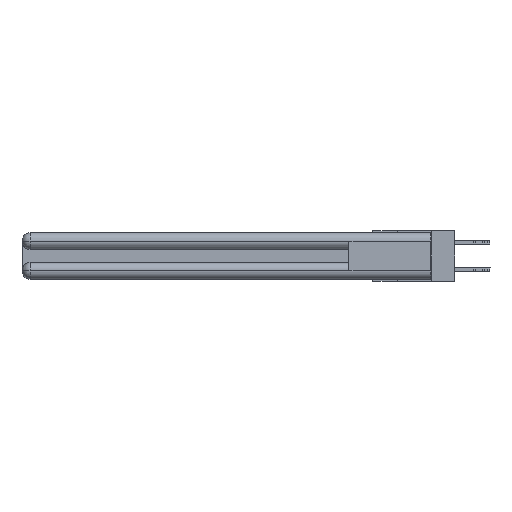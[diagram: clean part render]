
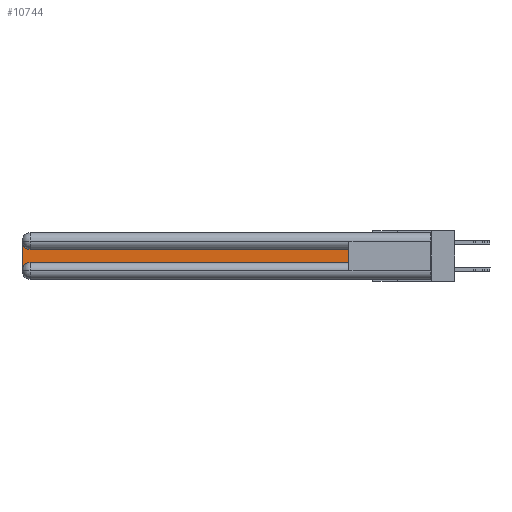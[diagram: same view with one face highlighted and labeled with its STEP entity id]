
A CAD part, left-side view. The second image highlights one B-rep face of the part: STEP entity #10744.
In plain terms, the highlighted planar face has unit normal (-1, 0, 0).
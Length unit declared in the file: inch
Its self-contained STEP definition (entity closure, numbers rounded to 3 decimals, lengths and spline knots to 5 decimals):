
#117 = LINE ( 'NONE', #29472, #9427 ) ;
#450 = EDGE_CURVE ( 'NONE', #2568, #6874, #19556, .T. ) ;
#1510 = CARTESIAN_POINT ( 'NONE',  ( 0.075, 0.6, -0.1225 ) ) ;
#2568 = VERTEX_POINT ( 'NONE', #13594 ) ;
#2750 = EDGE_LOOP ( 'NONE', ( #4872, #27061, #15855, #10406, #33133, #18451 ) ) ;
#3343 = DIRECTION ( 'NONE',  ( 0., -1., 0. ) ) ;
#4043 = DIRECTION ( 'NONE',  ( 1., 0., 0. ) ) ;
#4595 = AXIS2_PLACEMENT_3D ( 'NONE', #25945, #9605, #12233 ) ;
#4872 = ORIENTED_EDGE ( 'NONE', *, *, #20003, .T. ) ;
#6542 = LINE ( 'NONE', #30513, #8259 ) ;
#6874 = VERTEX_POINT ( 'NONE', #16815 ) ;
#7396 = DIRECTION ( 'NONE',  ( 0., 1., 0. ) ) ;
#7665 = EDGE_CURVE ( 'NONE', #16599, #8257, #28926, .T. ) ;
#8257 = VERTEX_POINT ( 'NONE', #32859 ) ;
#8259 = VECTOR ( 'NONE', #3343, 39.37008 ) ;
#9315 = CARTESIAN_POINT ( 'NONE',  ( 0.075, 0.6, -0.2175 ) ) ;
#9427 = VECTOR ( 'NONE', #32226, 39.37008 ) ;
#9605 = DIRECTION ( 'NONE',  ( 1., 0., 0. ) ) ;
#10406 = ORIENTED_EDGE ( 'NONE', *, *, #450, .T. ) ;
#10744 = ADVANCED_FACE ( 'NONE', ( #15960 ), #17992, .F. ) ;
#11776 = DIRECTION ( 'NONE',  ( 0., 0., -1. ) ) ;
#12233 = DIRECTION ( 'NONE',  ( 0., 0., -1. ) ) ;
#13594 = CARTESIAN_POINT ( 'NONE',  ( 0.075, 3., -0.2775 ) ) ;
#15482 = VERTEX_POINT ( 'NONE', #1510 ) ;
#15855 = ORIENTED_EDGE ( 'NONE', *, *, #17200, .T. ) ;
#15960 = FACE_OUTER_BOUND ( 'NONE', #2750, .T. ) ;
#16599 = VERTEX_POINT ( 'NONE', #23460 ) ;
#16815 = CARTESIAN_POINT ( 'NONE',  ( 0.075, 2.94, -0.2175 ) ) ;
#17200 = EDGE_CURVE ( 'NONE', #8257, #2568, #117, .T. ) ;
#17992 = PLANE ( 'NONE',  #4595 ) ;
#18451 = ORIENTED_EDGE ( 'NONE', *, *, #21430, .T. ) ;
#19099 = VECTOR ( 'NONE', #22168, 39.37008 ) ;
#19441 = CARTESIAN_POINT ( 'NONE',  ( 0.075, 0.6, -0.2175 ) ) ;
#19556 = CIRCLE ( 'NONE', #26095, 0.06 ) ;
#20003 = EDGE_CURVE ( 'NONE', #15482, #16599, #27233, .T. ) ;
#20514 = CARTESIAN_POINT ( 'NONE',  ( 0.075, 2.94, -0.0625 ) ) ;
#21430 = EDGE_CURVE ( 'NONE', #29503, #15482, #26272, .T. ) ;
#22168 = DIRECTION ( 'NONE',  ( 0., 0., 1. ) ) ;
#23002 = DIRECTION ( 'NONE',  ( 1., 0., 0. ) ) ;
#23460 = CARTESIAN_POINT ( 'NONE',  ( 0.075, 2.94, -0.1225 ) ) ;
#25945 = CARTESIAN_POINT ( 'NONE',  ( 0.075, 3., -0.1225 ) ) ;
#26095 = AXIS2_PLACEMENT_3D ( 'NONE', #33731, #23002, #11776 ) ;
#26272 = LINE ( 'NONE', #19441, #19099 ) ;
#26585 = CARTESIAN_POINT ( 'NONE',  ( 0.075, 0.6, -0.1225 ) ) ;
#27061 = ORIENTED_EDGE ( 'NONE', *, *, #7665, .T. ) ;
#27233 = LINE ( 'NONE', #26585, #27640 ) ;
#27608 = AXIS2_PLACEMENT_3D ( 'NONE', #20514, #4043, #28837 ) ;
#27640 = VECTOR ( 'NONE', #7396, 39.37008 ) ;
#28837 = DIRECTION ( 'NONE',  ( 0., 0., -1. ) ) ;
#28926 = CIRCLE ( 'NONE', #27608, 0.06 ) ;
#29472 = CARTESIAN_POINT ( 'NONE',  ( 0.075, 3., -0.2175 ) ) ;
#29503 = VERTEX_POINT ( 'NONE', #9315 ) ;
#30513 = CARTESIAN_POINT ( 'NONE',  ( 0.075, 0.6, -0.2175 ) ) ;
#31660 = EDGE_CURVE ( 'NONE', #6874, #29503, #6542, .T. ) ;
#32226 = DIRECTION ( 'NONE',  ( 0., 0., -1. ) ) ;
#32859 = CARTESIAN_POINT ( 'NONE',  ( 0.075, 3., -0.0625 ) ) ;
#33133 = ORIENTED_EDGE ( 'NONE', *, *, #31660, .T. ) ;
#33731 = CARTESIAN_POINT ( 'NONE',  ( 0.075, 2.94, -0.2775 ) ) ;
